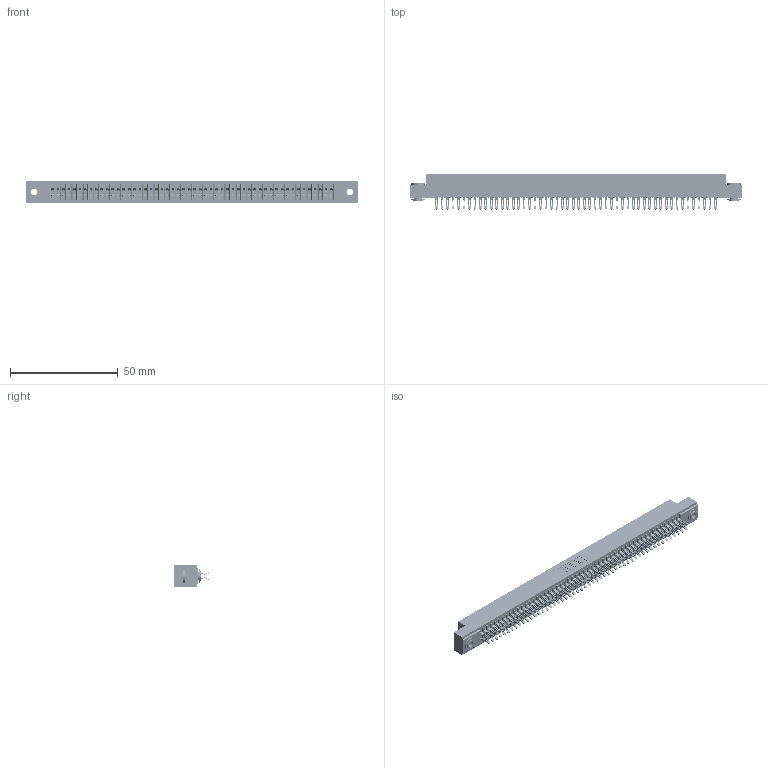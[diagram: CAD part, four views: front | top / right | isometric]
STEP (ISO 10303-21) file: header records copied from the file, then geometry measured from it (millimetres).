
FILE_DESCRIPTION (( 'STEP AP203' ), '1' );
FILE_NAME ('391-104-555-203.STEP', '2018-08-09T20:26:49', ( '' ), ( '' ), 'SwSTEP 2.0', 'SolidWorks 2016', '' );
FILE_SCHEMA (( 'CONFIG_CONTROL_DESIGN' ));
Length unit declared in the file: inch
Products named in the file (4): 391-104-555-203; 341 Part_.156 (3.96) Dia Mounting Holes; 341-292-001_341-292-155; 345-250-002_345-250-002-102
Assembly tree (107 placements, depth 2):
  391-104-555-203
    341 Part_.156 (3.96) Dia Mounting Holes
    341-292-001_341-292-155  x104
    345-250-002_345-250-002-102  x2
Bounding box: 154.31 x 16.31 x 10.16 mm (x, y, z)
Volume: 11537 mm3; surface area: 21888.3 mm2
Topology: 107 solids, 107 shells, 8280 faces, 24712 edges, 16086 vertices
Faces by surface type: plane 4460, cylinder 3604, sphere 106, torus 102, cone 8
Entity records: 63134 total; most frequent: CARTESIAN_POINT 10491, ORIENTED_EDGE 10408, DIRECTION 10180, EDGE_CURVE 5204, VECTOR 4190, LINE 4190, VERTEX_POINT 3290, AXIS2_PLACEMENT_3D 2995
